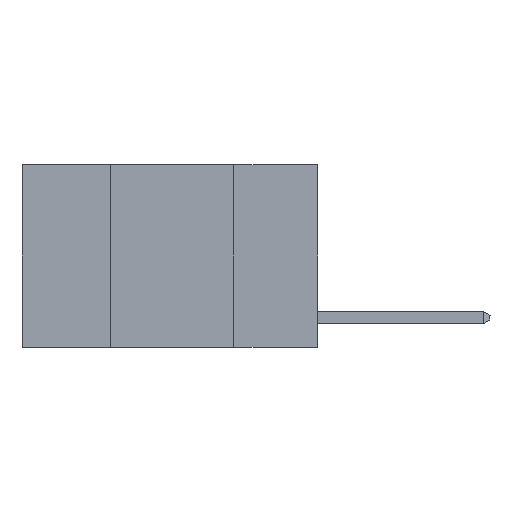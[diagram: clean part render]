
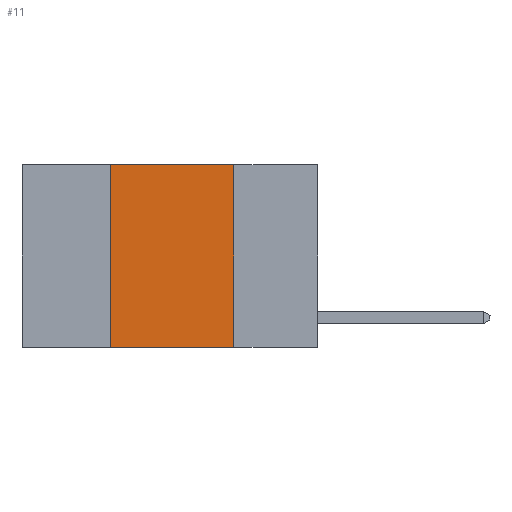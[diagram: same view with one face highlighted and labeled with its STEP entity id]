
A CAD part, left-side view. The second image highlights one B-rep face of the part: STEP entity #11.
In plain terms, the highlighted planar face has unit normal (-1, 0, 0).
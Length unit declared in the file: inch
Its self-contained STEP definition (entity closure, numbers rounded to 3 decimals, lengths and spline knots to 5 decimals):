
#11 = ADVANCED_FACE ( 'NONE', ( #2820 ), #17794, .F. ) ;
#552 = CARTESIAN_POINT ( 'NONE',  ( 0., 0.6, -0.37 ) ) ;
#953 = AXIS2_PLACEMENT_3D ( 'NONE', #7686, #3223, #12079 ) ;
#1150 = VECTOR ( 'NONE', #17126, 39.37008 ) ;
#1719 = LINE ( 'NONE', #552, #1150 ) ;
#1912 = VERTEX_POINT ( 'NONE', #11317 ) ;
#2086 = EDGE_CURVE ( 'NONE', #1912, #13089, #4216, .T. ) ;
#2820 = FACE_OUTER_BOUND ( 'NONE', #10936, .T. ) ;
#3223 = DIRECTION ( 'NONE',  ( 1., 0., 0. ) ) ;
#3629 = VECTOR ( 'NONE', #19546, 39.37008 ) ;
#4216 = LINE ( 'NONE', #9399, #22600 ) ;
#6650 = CARTESIAN_POINT ( 'NONE',  ( 0., 0.42, 0. ) ) ;
#6746 = ORIENTED_EDGE ( 'NONE', *, *, #15215, .F. ) ;
#7376 = VERTEX_POINT ( 'NONE', #23715 ) ;
#7686 = CARTESIAN_POINT ( 'NONE',  ( 0., 0.6, 0. ) ) ;
#7910 = LINE ( 'NONE', #6650, #3629 ) ;
#8191 = CARTESIAN_POINT ( 'NONE',  ( 0., 0.17, 0. ) ) ;
#9399 = CARTESIAN_POINT ( 'NONE',  ( 0., 0.6, 0. ) ) ;
#10475 = ORIENTED_EDGE ( 'NONE', *, *, #13247, .F. ) ;
#10936 = EDGE_LOOP ( 'NONE', ( #10475, #19163, #6746, #20599 ) ) ;
#11267 = DIRECTION ( 'NONE',  ( 0., -1., 0. ) ) ;
#11317 = CARTESIAN_POINT ( 'NONE',  ( 0., 0.42, 0. ) ) ;
#12011 = CARTESIAN_POINT ( 'NONE',  ( 0., 0.42, -0.37 ) ) ;
#12079 = DIRECTION ( 'NONE',  ( 0., 0., -1. ) ) ;
#13089 = VERTEX_POINT ( 'NONE', #17016 ) ;
#13247 = EDGE_CURVE ( 'NONE', #13089, #7376, #16990, .T. ) ;
#15215 = EDGE_CURVE ( 'NONE', #21980, #1912, #7910, .T. ) ;
#16405 = VECTOR ( 'NONE', #17430, 39.37008 ) ;
#16990 = LINE ( 'NONE', #8191, #16405 ) ;
#17016 = CARTESIAN_POINT ( 'NONE',  ( 0., 0.17, 0. ) ) ;
#17126 = DIRECTION ( 'NONE',  ( 0., -1., 0. ) ) ;
#17430 = DIRECTION ( 'NONE',  ( 0., 0., -1. ) ) ;
#17794 = PLANE ( 'NONE',  #953 ) ;
#18176 = EDGE_CURVE ( 'NONE', #21980, #7376, #1719, .T. ) ;
#19163 = ORIENTED_EDGE ( 'NONE', *, *, #2086, .F. ) ;
#19546 = DIRECTION ( 'NONE',  ( 0., 0., 1. ) ) ;
#20599 = ORIENTED_EDGE ( 'NONE', *, *, #18176, .T. ) ;
#21980 = VERTEX_POINT ( 'NONE', #12011 ) ;
#22600 = VECTOR ( 'NONE', #11267, 39.37008 ) ;
#23715 = CARTESIAN_POINT ( 'NONE',  ( 0., 0.17, -0.37 ) ) ;
